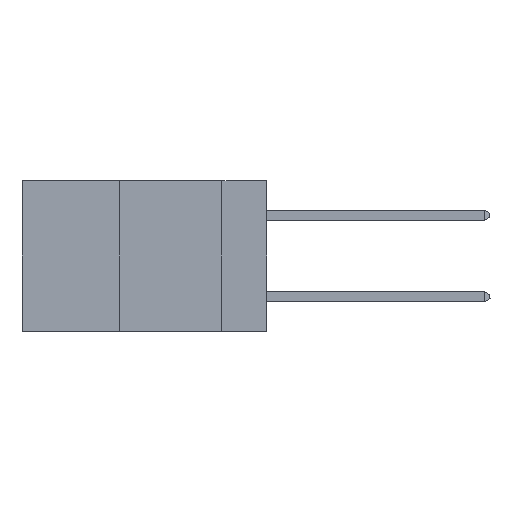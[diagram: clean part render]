
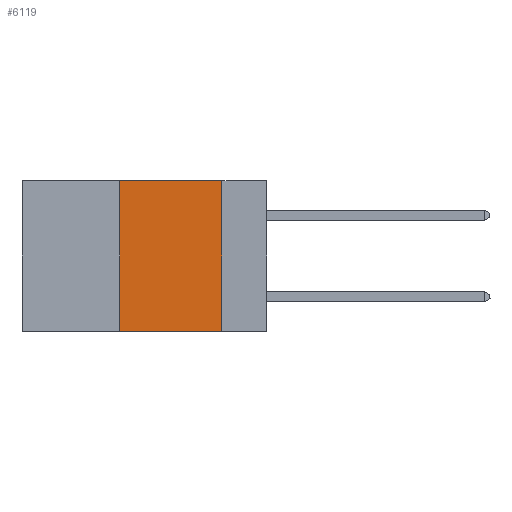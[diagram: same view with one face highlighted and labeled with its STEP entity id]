
A CAD part, left-side view. The second image highlights one B-rep face of the part: STEP entity #6119.
In plain terms, the highlighted planar face has unit normal (-1, 0, 0).
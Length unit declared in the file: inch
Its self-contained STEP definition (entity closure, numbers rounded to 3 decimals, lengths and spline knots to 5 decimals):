
#633 = EDGE_LOOP ( 'NONE', ( #4017, #9664, #18021, #8711 ) ) ;
#889 = VERTEX_POINT ( 'NONE', #14963 ) ;
#996 = VERTEX_POINT ( 'NONE', #3907 ) ;
#1301 = LINE ( 'NONE', #2946, #4827 ) ;
#1471 = CARTESIAN_POINT ( 'NONE',  ( 0., 0.36, 0. ) ) ;
#2030 = AXIS2_PLACEMENT_3D ( 'NONE', #2869, #13398, #4386 ) ;
#2725 = EDGE_CURVE ( 'NONE', #18178, #16553, #11445, .T. ) ;
#2758 = LINE ( 'NONE', #1471, #14270 ) ;
#2869 = CARTESIAN_POINT ( 'NONE',  ( 0., 0.6, 0. ) ) ;
#2946 = CARTESIAN_POINT ( 'NONE',  ( 0., 0.6, -0.37 ) ) ;
#3907 = CARTESIAN_POINT ( 'NONE',  ( 0., 0.36, 0. ) ) ;
#4009 = EDGE_CURVE ( 'NONE', #889, #16553, #1301, .T. ) ;
#4017 = ORIENTED_EDGE ( 'NONE', *, *, #2725, .F. ) ;
#4386 = DIRECTION ( 'NONE',  ( 0., 0., -1. ) ) ;
#4448 = CARTESIAN_POINT ( 'NONE',  ( 0., 0.6, 0. ) ) ;
#4827 = VECTOR ( 'NONE', #14973, 39.37008 ) ;
#6119 = ADVANCED_FACE ( 'NONE', ( #14192 ), #19374, .F. ) ;
#7956 = VECTOR ( 'NONE', #9712, 39.37008 ) ;
#8711 = ORIENTED_EDGE ( 'NONE', *, *, #4009, .T. ) ;
#9425 = CARTESIAN_POINT ( 'NONE',  ( 0., 0.11, -0.37 ) ) ;
#9662 = VECTOR ( 'NONE', #13465, 39.37008 ) ;
#9664 = ORIENTED_EDGE ( 'NONE', *, *, #15667, .F. ) ;
#9712 = DIRECTION ( 'NONE',  ( 0., 0., -1. ) ) ;
#11318 = EDGE_CURVE ( 'NONE', #889, #996, #2758, .T. ) ;
#11445 = LINE ( 'NONE', #18204, #7956 ) ;
#13398 = DIRECTION ( 'NONE',  ( 1., 0., 0. ) ) ;
#13465 = DIRECTION ( 'NONE',  ( 0., -1., 0. ) ) ;
#14136 = LINE ( 'NONE', #4448, #9662 ) ;
#14192 = FACE_OUTER_BOUND ( 'NONE', #633, .T. ) ;
#14211 = CARTESIAN_POINT ( 'NONE',  ( 0., 0.11, 0. ) ) ;
#14270 = VECTOR ( 'NONE', #16486, 39.37008 ) ;
#14963 = CARTESIAN_POINT ( 'NONE',  ( 0., 0.36, -0.37 ) ) ;
#14973 = DIRECTION ( 'NONE',  ( 0., -1., 0. ) ) ;
#15667 = EDGE_CURVE ( 'NONE', #996, #18178, #14136, .T. ) ;
#16486 = DIRECTION ( 'NONE',  ( 0., 0., 1. ) ) ;
#16553 = VERTEX_POINT ( 'NONE', #9425 ) ;
#18021 = ORIENTED_EDGE ( 'NONE', *, *, #11318, .F. ) ;
#18178 = VERTEX_POINT ( 'NONE', #14211 ) ;
#18204 = CARTESIAN_POINT ( 'NONE',  ( 0., 0.11, 0. ) ) ;
#19374 = PLANE ( 'NONE',  #2030 ) ;
